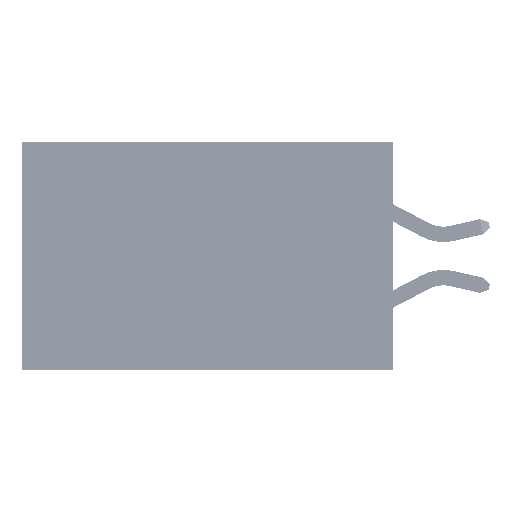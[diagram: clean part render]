
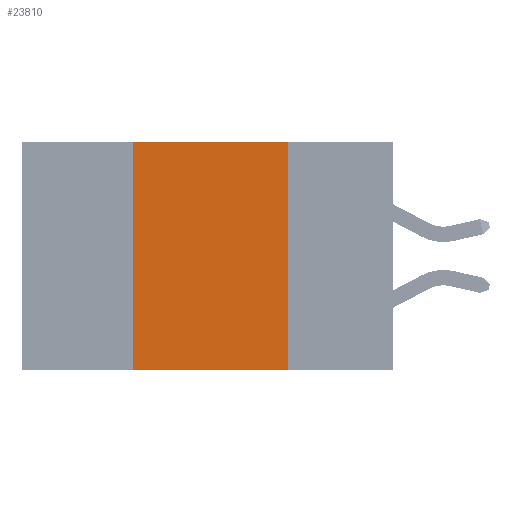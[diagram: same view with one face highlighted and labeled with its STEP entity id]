
A CAD part, left-side view. The second image highlights one B-rep face of the part: STEP entity #23810.
In plain terms, the highlighted planar face has unit normal (-1, 0, 0).
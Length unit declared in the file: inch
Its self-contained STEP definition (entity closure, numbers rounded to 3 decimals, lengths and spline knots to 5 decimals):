
#380 = EDGE_CURVE ( 'NONE', #36881, #44930, #14633, .T. ) ;
#456 = FACE_OUTER_BOUND ( 'NONE', #47481, .T. ) ;
#496 = VECTOR ( 'NONE', #32463, 39.37008 ) ;
#2049 = LINE ( 'NONE', #35867, #30976 ) ;
#3241 = ORIENTED_EDGE ( 'NONE', *, *, #380, .F. ) ;
#3993 = CARTESIAN_POINT ( 'NONE',  ( 0., 0.6, 0. ) ) ;
#4706 = CARTESIAN_POINT ( 'NONE',  ( 0., 0.17, 0. ) ) ;
#10804 = EDGE_CURVE ( 'NONE', #48539, #49391, #19916, .T. ) ;
#11921 = VECTOR ( 'NONE', #15468, 39.37008 ) ;
#12331 = ORIENTED_EDGE ( 'NONE', *, *, #10804, .F. ) ;
#14633 = LINE ( 'NONE', #4706, #496 ) ;
#15468 = DIRECTION ( 'NONE',  ( 0., 0., 1. ) ) ;
#15525 = DIRECTION ( 'NONE',  ( 0., -1., 0. ) ) ;
#17143 = DIRECTION ( 'NONE',  ( 1., 0., 0. ) ) ;
#17662 = DIRECTION ( 'NONE',  ( 0., 0., -1. ) ) ;
#19058 = CARTESIAN_POINT ( 'NONE',  ( 0., 0.42, -0.37 ) ) ;
#19916 = LINE ( 'NONE', #50229, #11921 ) ;
#21192 = LINE ( 'NONE', #3993, #39639 ) ;
#23810 = ADVANCED_FACE ( 'NONE', ( #456 ), #33030, .F. ) ;
#25684 = CARTESIAN_POINT ( 'NONE',  ( 0., 0.17, 0. ) ) ;
#28493 = DIRECTION ( 'NONE',  ( 0., -1., 0. ) ) ;
#30976 = VECTOR ( 'NONE', #28493, 39.37008 ) ;
#31410 = AXIS2_PLACEMENT_3D ( 'NONE', #41429, #17143, #17662 ) ;
#32463 = DIRECTION ( 'NONE',  ( 0., 0., -1. ) ) ;
#33030 = PLANE ( 'NONE',  #31410 ) ;
#35867 = CARTESIAN_POINT ( 'NONE',  ( 0., 0.6, -0.37 ) ) ;
#36881 = VERTEX_POINT ( 'NONE', #25684 ) ;
#38243 = ORIENTED_EDGE ( 'NONE', *, *, #39944, .F. ) ;
#39623 = CARTESIAN_POINT ( 'NONE',  ( 0., 0.42, 0. ) ) ;
#39639 = VECTOR ( 'NONE', #15525, 39.37008 ) ;
#39944 = EDGE_CURVE ( 'NONE', #49391, #36881, #21192, .T. ) ;
#41429 = CARTESIAN_POINT ( 'NONE',  ( 0., 0.6, 0. ) ) ;
#43977 = EDGE_CURVE ( 'NONE', #48539, #44930, #2049, .T. ) ;
#44930 = VERTEX_POINT ( 'NONE', #48749 ) ;
#47481 = EDGE_LOOP ( 'NONE', ( #3241, #38243, #12331, #49236 ) ) ;
#48539 = VERTEX_POINT ( 'NONE', #19058 ) ;
#48749 = CARTESIAN_POINT ( 'NONE',  ( 0., 0.17, -0.37 ) ) ;
#49236 = ORIENTED_EDGE ( 'NONE', *, *, #43977, .T. ) ;
#49391 = VERTEX_POINT ( 'NONE', #39623 ) ;
#50229 = CARTESIAN_POINT ( 'NONE',  ( 0., 0.42, 0. ) ) ;
